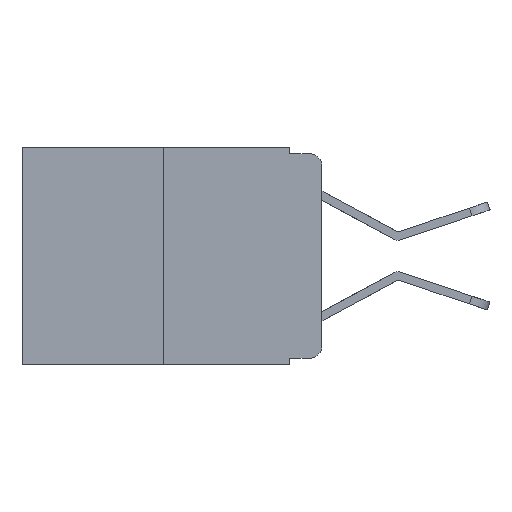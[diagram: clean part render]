
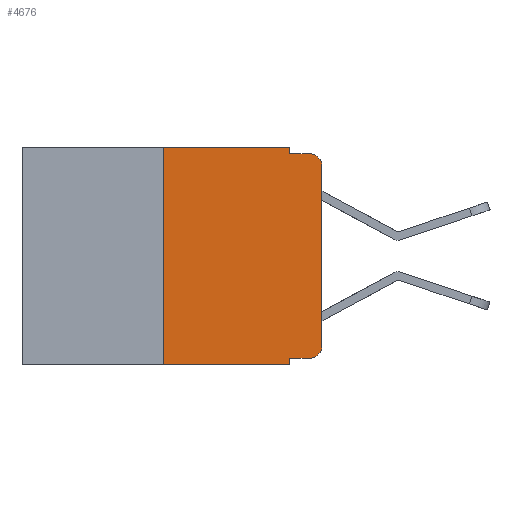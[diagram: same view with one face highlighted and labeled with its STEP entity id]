
A CAD part, left-side view. The second image highlights one B-rep face of the part: STEP entity #4676.
In plain terms, the highlighted planar face has unit normal (-1, 0, 0).
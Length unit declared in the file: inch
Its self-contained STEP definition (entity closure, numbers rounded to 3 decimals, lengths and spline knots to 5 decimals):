
#170 = CIRCLE ( 'NONE', #5904, 0.02 ) ;
#352 = CARTESIAN_POINT ( 'NONE',  ( 0., 0.25, -0.343 ) ) ;
#368 = VERTEX_POINT ( 'NONE', #9189 ) ;
#374 = CARTESIAN_POINT ( 'NONE',  ( 0., 0.051, -0.333 ) ) ;
#470 = ORIENTED_EDGE ( 'NONE', *, *, #12074, .T. ) ;
#573 = DIRECTION ( 'NONE',  ( -1., 0., 0. ) ) ;
#602 = ORIENTED_EDGE ( 'NONE', *, *, #11496, .T. ) ;
#622 = CARTESIAN_POINT ( 'NONE',  ( 0., 0.051, -0.01 ) ) ;
#691 = ORIENTED_EDGE ( 'NONE', *, *, #10328, .F. ) ;
#1043 = ORIENTED_EDGE ( 'NONE', *, *, #9738, .F. ) ;
#1063 = DIRECTION ( 'NONE',  ( 0., 0., -1. ) ) ;
#1065 = ORIENTED_EDGE ( 'NONE', *, *, #7812, .F. ) ;
#1210 = ORIENTED_EDGE ( 'NONE', *, *, #9117, .F. ) ;
#1226 = DIRECTION ( 'NONE',  ( 0., 0., 1. ) ) ;
#1247 = LINE ( 'NONE', #5927, #10760 ) ;
#1398 = DIRECTION ( 'NONE',  ( -1., 0., 0. ) ) ;
#1539 = ORIENTED_EDGE ( 'NONE', *, *, #6843, .T. ) ;
#1627 = LINE ( 'NONE', #5738, #11090 ) ;
#1806 = VERTEX_POINT ( 'NONE', #352 ) ;
#1810 = ORIENTED_EDGE ( 'NONE', *, *, #8500, .F. ) ;
#1914 = VECTOR ( 'NONE', #8584, 39.37008 ) ;
#2057 = VECTOR ( 'NONE', #1063, 39.37008 ) ;
#2100 = CARTESIAN_POINT ( 'NONE',  ( 0., 0., -0.313 ) ) ;
#2284 = ORIENTED_EDGE ( 'NONE', *, *, #7308, .T. ) ;
#2359 = LINE ( 'NONE', #6976, #2057 ) ;
#2434 = ORIENTED_EDGE ( 'NONE', *, *, #6684, .T. ) ;
#2564 = CIRCLE ( 'NONE', #7012, 0.02 ) ;
#3339 = VERTEX_POINT ( 'NONE', #10068 ) ;
#3870 = FACE_OUTER_BOUND ( 'NONE', #4301, .T. ) ;
#3880 = CARTESIAN_POINT ( 'NONE',  ( 0., 0.473, 0. ) ) ;
#3941 = PLANE ( 'NONE',  #4021 ) ;
#4021 = AXIS2_PLACEMENT_3D ( 'NONE', #4950, #11330, #5909 ) ;
#4237 = CARTESIAN_POINT ( 'NONE',  ( 0., 0.25, 0. ) ) ;
#4301 = EDGE_LOOP ( 'NONE', ( #470, #602, #691, #1043, #1065, #1210, #1539, #1810, #2284, #2434 ) ) ;
#4613 = LINE ( 'NONE', #3880, #1914 ) ;
#4626 = VECTOR ( 'NONE', #10757, 39.37008 ) ;
#4676 = ADVANCED_FACE ( 'NONE', ( #3870 ), #3941, .F. ) ;
#4950 = CARTESIAN_POINT ( 'NONE',  ( 0., 0.473, 0. ) ) ;
#5245 = LINE ( 'NONE', #5288, #4626 ) ;
#5288 = CARTESIAN_POINT ( 'NONE',  ( 0., 0.051, -0.333 ) ) ;
#5315 = VECTOR ( 'NONE', #9322, 39.37008 ) ;
#5738 = CARTESIAN_POINT ( 'NONE',  ( 0., 0.473, -0.343 ) ) ;
#5742 = VERTEX_POINT ( 'NONE', #11681 ) ;
#5904 = AXIS2_PLACEMENT_3D ( 'NONE', #6533, #573, #7478 ) ;
#5909 = DIRECTION ( 'NONE',  ( 0., 0., -1. ) ) ;
#5927 = CARTESIAN_POINT ( 'NONE',  ( 0., 0.051, 0. ) ) ;
#6533 = CARTESIAN_POINT ( 'NONE',  ( 0., 0.02, -0.313 ) ) ;
#6684 = EDGE_CURVE ( 'NONE', #7743, #9007, #170, .T. ) ;
#6702 = DIRECTION ( 'NONE',  ( 0., -1., 0. ) ) ;
#6843 = EDGE_CURVE ( 'NONE', #1806, #6962, #1627, .T. ) ;
#6962 = VERTEX_POINT ( 'NONE', #12165 ) ;
#6976 = CARTESIAN_POINT ( 'NONE',  ( 0., 0.051, 0. ) ) ;
#7012 = AXIS2_PLACEMENT_3D ( 'NONE', #7298, #1398, #8198 ) ;
#7036 = CARTESIAN_POINT ( 'NONE',  ( 0., 0., 0. ) ) ;
#7201 = CARTESIAN_POINT ( 'NONE',  ( 0., 0., -0.03 ) ) ;
#7298 = CARTESIAN_POINT ( 'NONE',  ( 0., 0.02, -0.03 ) ) ;
#7308 = EDGE_CURVE ( 'NONE', #7437, #7743, #5245, .T. ) ;
#7437 = VERTEX_POINT ( 'NONE', #374 ) ;
#7478 = DIRECTION ( 'NONE',  ( 0., 0., -1. ) ) ;
#7743 = VERTEX_POINT ( 'NONE', #12034 ) ;
#7812 = EDGE_CURVE ( 'NONE', #8539, #368, #4613, .T. ) ;
#7818 = LINE ( 'NONE', #622, #5315 ) ;
#8198 = DIRECTION ( 'NONE',  ( 0., 0., -1. ) ) ;
#8500 = EDGE_CURVE ( 'NONE', #7437, #6962, #2359, .T. ) ;
#8539 = VERTEX_POINT ( 'NONE', #10644 ) ;
#8584 = DIRECTION ( 'NONE',  ( 0., -1., 0. ) ) ;
#8941 = VECTOR ( 'NONE', #1226, 39.37008 ) ;
#9007 = VERTEX_POINT ( 'NONE', #2100 ) ;
#9117 = EDGE_CURVE ( 'NONE', #1806, #8539, #11318, .T. ) ;
#9189 = CARTESIAN_POINT ( 'NONE',  ( 0., 0.051, 0. ) ) ;
#9322 = DIRECTION ( 'NONE',  ( 0., -1., 0. ) ) ;
#9738 = EDGE_CURVE ( 'NONE', #368, #5742, #1247, .T. ) ;
#10068 = CARTESIAN_POINT ( 'NONE',  ( 0., 0.02, -0.01 ) ) ;
#10132 = LINE ( 'NONE', #7036, #11623 ) ;
#10328 = EDGE_CURVE ( 'NONE', #5742, #3339, #7818, .T. ) ;
#10644 = CARTESIAN_POINT ( 'NONE',  ( 0., 0.25, 0. ) ) ;
#10757 = DIRECTION ( 'NONE',  ( 0., -1., 0. ) ) ;
#10760 = VECTOR ( 'NONE', #11311, 39.37008 ) ;
#11090 = VECTOR ( 'NONE', #6702, 39.37008 ) ;
#11311 = DIRECTION ( 'NONE',  ( 0., 0., -1. ) ) ;
#11318 = LINE ( 'NONE', #4237, #8941 ) ;
#11330 = DIRECTION ( 'NONE',  ( 1., 0., 0. ) ) ;
#11496 = EDGE_CURVE ( 'NONE', #12240, #3339, #2564, .T. ) ;
#11506 = DIRECTION ( 'NONE',  ( 0., 0., 1. ) ) ;
#11623 = VECTOR ( 'NONE', #11506, 39.37008 ) ;
#11681 = CARTESIAN_POINT ( 'NONE',  ( 0., 0.051, -0.01 ) ) ;
#12034 = CARTESIAN_POINT ( 'NONE',  ( 0., 0.02, -0.333 ) ) ;
#12074 = EDGE_CURVE ( 'NONE', #9007, #12240, #10132, .T. ) ;
#12165 = CARTESIAN_POINT ( 'NONE',  ( 0., 0.051, -0.343 ) ) ;
#12240 = VERTEX_POINT ( 'NONE', #7201 ) ;
